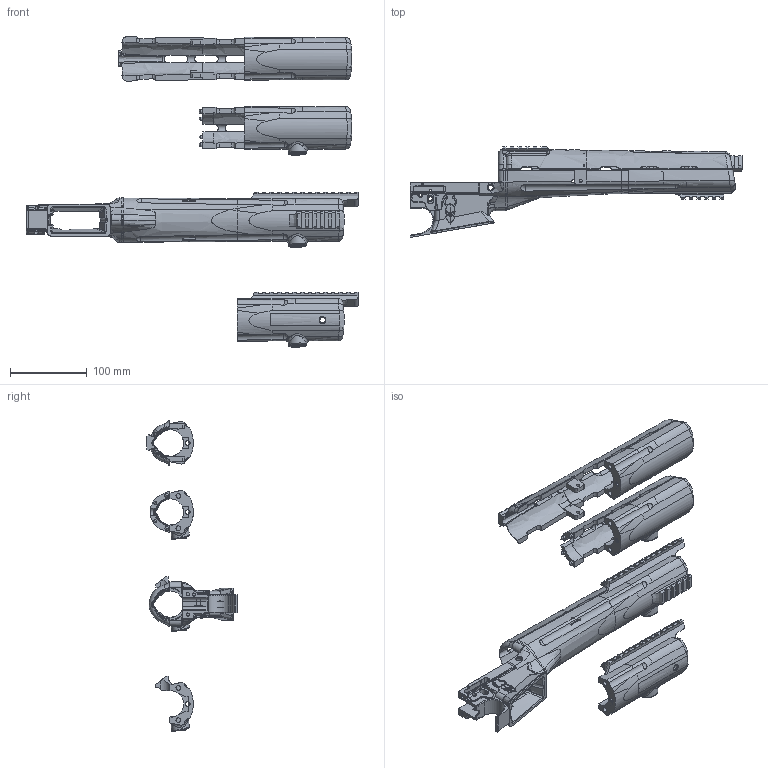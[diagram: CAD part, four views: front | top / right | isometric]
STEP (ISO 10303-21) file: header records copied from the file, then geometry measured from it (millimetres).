
FILE_DESCRIPTION(/* description */ (''),/* implementation_level */ '2;1');
FILE_NAME(/* name */ 'AA3 v8.step',/* time_stamp */ '2020-05-20T22:27:36-05:00',/* author */ (''),/* organization */ (''),/* preprocessor_version */ 'ST-DEVELOPER v18.1',/* originating_system */ 'Autodesk Translation Framework v9.3.0.1241',/* authorisation */ '');
FILE_SCHEMA (('AUTOMOTIVE_DESIGN { 1 0 10303 214 3 1 1 }'));
Length unit declared in the file: millimetre
Products named in the file (1): AA3
Bounding box: 432.4 x 117.85 x 404.41 mm (x, y, z)
Volume: 996934.5 mm3; surface area: 317947.7 mm2
Topology: 11 solids, 11 shells, 1732 faces, 4848 edges, 3176 vertices
Faces by surface type: plane 773, bspline 539, cylinder 342, torus 55, sphere 21, cone 2
Full cylindrical faces by diameter (mm): 2 x2, 2.103 x3, 2.362 x2, 3.962 x2, 3.969 x1, 4 x25, 4.9 x3, 5 x10, 5.182 x1, 5.389 x1, 5.394 x1, 6 x23, 6.375 x2, 7 x1, 7.938 x1, 8.895 x1, 13 x3, 23.283 x3
Entity records: 79361 total; most frequent: CARTESIAN_POINT 39424, ORIENTED_EDGE 9658, DIRECTION 6162, EDGE_CURVE 4829, VERTEX_POINT 3176, LINE 2270, VECTOR 2270, AXIS2_PLACEMENT_3D 1946
